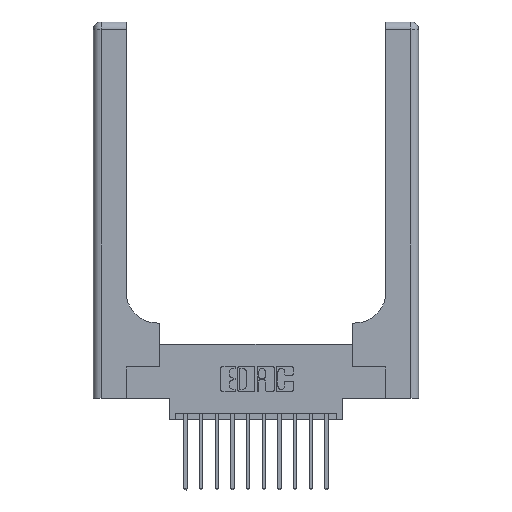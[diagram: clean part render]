
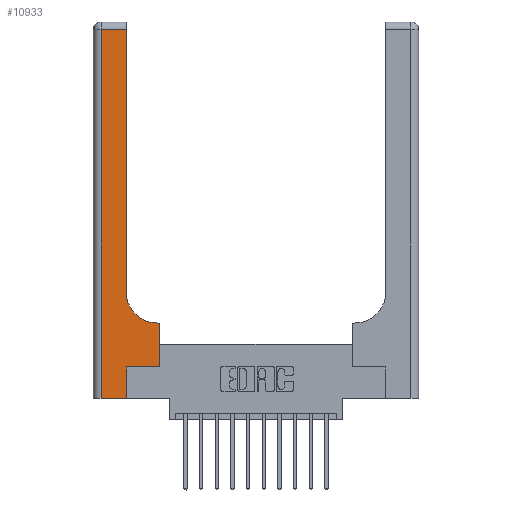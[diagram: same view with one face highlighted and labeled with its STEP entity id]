
A CAD part, top view. The second image highlights one B-rep face of the part: STEP entity #10933.
In plain terms, the highlighted planar face has unit normal (0, 0, 1).
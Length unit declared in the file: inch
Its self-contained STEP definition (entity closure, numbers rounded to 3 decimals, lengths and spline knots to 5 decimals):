
#122 = VECTOR ( 'NONE', #12451, 39.37008 ) ;
#173 = DIRECTION ( 'NONE',  ( -1., 0., 0. ) ) ;
#654 = CARTESIAN_POINT ( 'NONE',  ( 0.06, 3., 0.37 ) ) ;
#995 = LINE ( 'NONE', #8625, #3941 ) ;
#1127 = CARTESIAN_POINT ( 'NONE',  ( 0.528, 0.25, 0.37 ) ) ;
#1180 = DIRECTION ( 'NONE',  ( 1., 0., 0. ) ) ;
#1233 = ORIENTED_EDGE ( 'NONE', *, *, #8346, .T. ) ;
#1352 = CARTESIAN_POINT ( 'NONE',  ( 0.528, 0.6, 0.37 ) ) ;
#1366 = EDGE_CURVE ( 'NONE', #7915, #14365, #4520, .T. ) ;
#1375 = LINE ( 'NONE', #15241, #2152 ) ;
#1566 = EDGE_CURVE ( 'NONE', #3325, #16127, #1375, .T. ) ;
#1832 = CARTESIAN_POINT ( 'NONE',  ( 0.26, 2.94, 0.37 ) ) ;
#2152 = VECTOR ( 'NONE', #9143, 39.37008 ) ;
#2178 = CARTESIAN_POINT ( 'NONE',  ( 0.51, 0.85, 0.37 ) ) ;
#2234 = EDGE_LOOP ( 'NONE', ( #10297, #14285, #1233, #9541, #4173, #14729, #8234, #5646, #14594 ) ) ;
#2241 = VECTOR ( 'NONE', #14066, 39.37008 ) ;
#2339 = CARTESIAN_POINT ( 'NONE',  ( 0.265, 0., 0.37 ) ) ;
#2487 = LINE ( 'NONE', #4555, #11741 ) ;
#2959 = LINE ( 'NONE', #654, #11445 ) ;
#3325 = VERTEX_POINT ( 'NONE', #7921 ) ;
#3444 = DIRECTION ( 'NONE',  ( 1., 0., 0. ) ) ;
#3741 = VECTOR ( 'NONE', #1180, 39.37008 ) ;
#3941 = VECTOR ( 'NONE', #6137, 39.37008 ) ;
#4173 = ORIENTED_EDGE ( 'NONE', *, *, #11916, .T. ) ;
#4520 = LINE ( 'NONE', #4915, #3741 ) ;
#4555 = CARTESIAN_POINT ( 'NONE',  ( 0.265, 0.25, 0.37 ) ) ;
#4915 = CARTESIAN_POINT ( 'NONE',  ( 0., 0., 0.37 ) ) ;
#5019 = EDGE_CURVE ( 'NONE', #16127, #7405, #15125, .T. ) ;
#5352 = VERTEX_POINT ( 'NONE', #7814 ) ;
#5361 = CARTESIAN_POINT ( 'NONE',  ( 0., 2.94, 0.37 ) ) ;
#5418 = CARTESIAN_POINT ( 'NONE',  ( 0.06, 2.94, 0.37 ) ) ;
#5646 = ORIENTED_EDGE ( 'NONE', *, *, #9433, .T. ) ;
#6137 = DIRECTION ( 'NONE',  ( 0., 1., 0. ) ) ;
#7405 = VERTEX_POINT ( 'NONE', #5418 ) ;
#7525 = VERTEX_POINT ( 'NONE', #15572 ) ;
#7770 = DIRECTION ( 'NONE',  ( 0., 0., -1. ) ) ;
#7814 = CARTESIAN_POINT ( 'NONE',  ( 0.528, 0.25, 0.37 ) ) ;
#7915 = VERTEX_POINT ( 'NONE', #8817 ) ;
#7921 = CARTESIAN_POINT ( 'NONE',  ( 0.26, 0.85, 0.37 ) ) ;
#8044 = VERTEX_POINT ( 'NONE', #13904 ) ;
#8234 = ORIENTED_EDGE ( 'NONE', *, *, #9814, .T. ) ;
#8346 = EDGE_CURVE ( 'NONE', #7405, #7915, #2959, .T. ) ;
#8625 = CARTESIAN_POINT ( 'NONE',  ( 0.265, 0., 0.37 ) ) ;
#8817 = CARTESIAN_POINT ( 'NONE',  ( 0.06, 0., 0.37 ) ) ;
#9075 = LINE ( 'NONE', #10469, #15197 ) ;
#9143 = DIRECTION ( 'NONE',  ( 0., 1., 0. ) ) ;
#9433 = EDGE_CURVE ( 'NONE', #14489, #7525, #9075, .T. ) ;
#9541 = ORIENTED_EDGE ( 'NONE', *, *, #1366, .T. ) ;
#9814 = EDGE_CURVE ( 'NONE', #5352, #14489, #13479, .T. ) ;
#9867 = AXIS2_PLACEMENT_3D ( 'NONE', #12720, #7770, #173 ) ;
#10297 = ORIENTED_EDGE ( 'NONE', *, *, #1566, .T. ) ;
#10469 = CARTESIAN_POINT ( 'NONE',  ( 0.26, 0.6, 0.37 ) ) ;
#10683 = EDGE_CURVE ( 'NONE', #8044, #5352, #2487, .T. ) ;
#10933 = ADVANCED_FACE ( 'NONE', ( #14772 ), #15154, .F. ) ;
#11033 = DIRECTION ( 'NONE',  ( 0., 0., -1. ) ) ;
#11445 = VECTOR ( 'NONE', #14427, 39.37008 ) ;
#11635 = AXIS2_PLACEMENT_3D ( 'NONE', #2178, #11033, #3444 ) ;
#11741 = VECTOR ( 'NONE', #14523, 39.37008 ) ;
#11755 = DIRECTION ( 'NONE',  ( -1., 0., 0. ) ) ;
#11916 = EDGE_CURVE ( 'NONE', #14365, #8044, #995, .T. ) ;
#12405 = EDGE_CURVE ( 'NONE', #7525, #3325, #13892, .T. ) ;
#12451 = DIRECTION ( 'NONE',  ( 0., 1., 0. ) ) ;
#12720 = CARTESIAN_POINT ( 'NONE',  ( 0., 3., 0.37 ) ) ;
#13479 = LINE ( 'NONE', #1127, #122 ) ;
#13892 = CIRCLE ( 'NONE', #11635, 0.25 ) ;
#13904 = CARTESIAN_POINT ( 'NONE',  ( 0.265, 0.25, 0.37 ) ) ;
#14066 = DIRECTION ( 'NONE',  ( -1., 0., 0. ) ) ;
#14285 = ORIENTED_EDGE ( 'NONE', *, *, #5019, .T. ) ;
#14365 = VERTEX_POINT ( 'NONE', #2339 ) ;
#14427 = DIRECTION ( 'NONE',  ( 0., -1., 0. ) ) ;
#14489 = VERTEX_POINT ( 'NONE', #1352 ) ;
#14523 = DIRECTION ( 'NONE',  ( 1., 0., 0. ) ) ;
#14594 = ORIENTED_EDGE ( 'NONE', *, *, #12405, .T. ) ;
#14729 = ORIENTED_EDGE ( 'NONE', *, *, #10683, .T. ) ;
#14772 = FACE_OUTER_BOUND ( 'NONE', #2234, .T. ) ;
#15125 = LINE ( 'NONE', #5361, #2241 ) ;
#15154 = PLANE ( 'NONE',  #9867 ) ;
#15197 = VECTOR ( 'NONE', #11755, 39.37008 ) ;
#15241 = CARTESIAN_POINT ( 'NONE',  ( 0.26, 3., 0.37 ) ) ;
#15572 = CARTESIAN_POINT ( 'NONE',  ( 0.51, 0.6, 0.37 ) ) ;
#16127 = VERTEX_POINT ( 'NONE', #1832 ) ;
